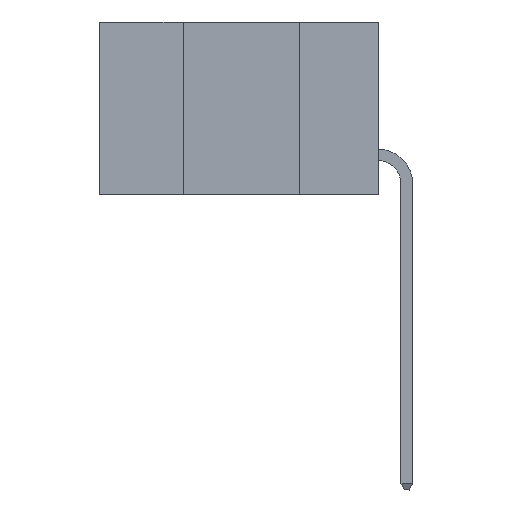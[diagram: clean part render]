
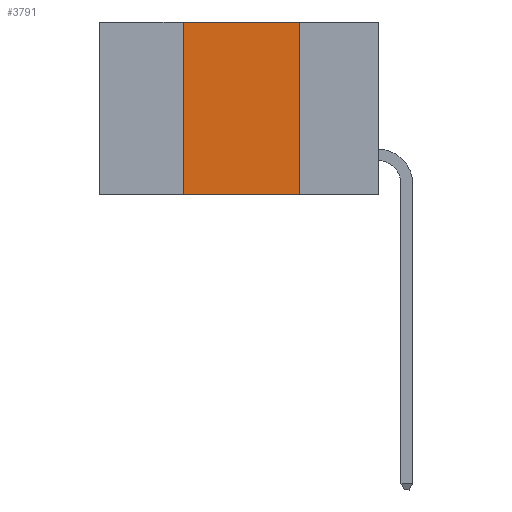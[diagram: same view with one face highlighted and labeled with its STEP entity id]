
A CAD part, left-side view. The second image highlights one B-rep face of the part: STEP entity #3791.
In plain terms, the highlighted planar face has unit normal (-1, 0, 0).
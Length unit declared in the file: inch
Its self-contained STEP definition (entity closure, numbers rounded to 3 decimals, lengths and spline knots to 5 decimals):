
#99 = VECTOR ( 'NONE', #8185, 39.37008 ) ;
#192 = CARTESIAN_POINT ( 'NONE',  ( 0., 0.6, 0. ) ) ;
#421 = VECTOR ( 'NONE', #9140, 39.37008 ) ;
#573 = CARTESIAN_POINT ( 'NONE',  ( 0., 0.6, 0. ) ) ;
#913 = LINE ( 'NONE', #4897, #99 ) ;
#1423 = DIRECTION ( 'NONE',  ( 0., 0., -1. ) ) ;
#2024 = CARTESIAN_POINT ( 'NONE',  ( 0., 0.42, -0.37 ) ) ;
#2042 = VERTEX_POINT ( 'NONE', #2024 ) ;
#2150 = ORIENTED_EDGE ( 'NONE', *, *, #2958, .F. ) ;
#2161 = VERTEX_POINT ( 'NONE', #8413 ) ;
#2257 = DIRECTION ( 'NONE',  ( 0., 0., -1. ) ) ;
#2400 = ORIENTED_EDGE ( 'NONE', *, *, #9526, .F. ) ;
#2404 = ORIENTED_EDGE ( 'NONE', *, *, #5652, .F. ) ;
#2718 = LINE ( 'NONE', #3962, #421 ) ;
#2752 = CARTESIAN_POINT ( 'NONE',  ( 0., 0.17, -0.37 ) ) ;
#2958 = EDGE_CURVE ( 'NONE', #2161, #3623, #4006, .T. ) ;
#3623 = VERTEX_POINT ( 'NONE', #2752 ) ;
#3791 = ADVANCED_FACE ( 'NONE', ( #5563 ), #7113, .F. ) ;
#3962 = CARTESIAN_POINT ( 'NONE',  ( 0., 0.6, -0.37 ) ) ;
#4006 = LINE ( 'NONE', #10372, #9569 ) ;
#4219 = ORIENTED_EDGE ( 'NONE', *, *, #4382, .T. ) ;
#4382 = EDGE_CURVE ( 'NONE', #2042, #3623, #2718, .T. ) ;
#4897 = CARTESIAN_POINT ( 'NONE',  ( 0., 0.42, -0.37 ) ) ;
#5114 = EDGE_LOOP ( 'NONE', ( #2150, #2400, #2404, #4219 ) ) ;
#5548 = VERTEX_POINT ( 'NONE', #9547 ) ;
#5563 = FACE_OUTER_BOUND ( 'NONE', #5114, .T. ) ;
#5652 = EDGE_CURVE ( 'NONE', #2042, #5548, #913, .T. ) ;
#5917 = LINE ( 'NONE', #192, #10292 ) ;
#6603 = DIRECTION ( 'NONE',  ( 0., -1., 0. ) ) ;
#7113 = PLANE ( 'NONE',  #8742 ) ;
#8185 = DIRECTION ( 'NONE',  ( 0., 0., 1. ) ) ;
#8413 = CARTESIAN_POINT ( 'NONE',  ( 0., 0.17, 0. ) ) ;
#8707 = DIRECTION ( 'NONE',  ( 1., 0., 0. ) ) ;
#8742 = AXIS2_PLACEMENT_3D ( 'NONE', #573, #8707, #1423 ) ;
#9140 = DIRECTION ( 'NONE',  ( 0., -1., 0. ) ) ;
#9526 = EDGE_CURVE ( 'NONE', #5548, #2161, #5917, .T. ) ;
#9547 = CARTESIAN_POINT ( 'NONE',  ( 0., 0.42, 0. ) ) ;
#9569 = VECTOR ( 'NONE', #2257, 39.37008 ) ;
#10292 = VECTOR ( 'NONE', #6603, 39.37008 ) ;
#10372 = CARTESIAN_POINT ( 'NONE',  ( 0., 0.17, -0.37 ) ) ;
